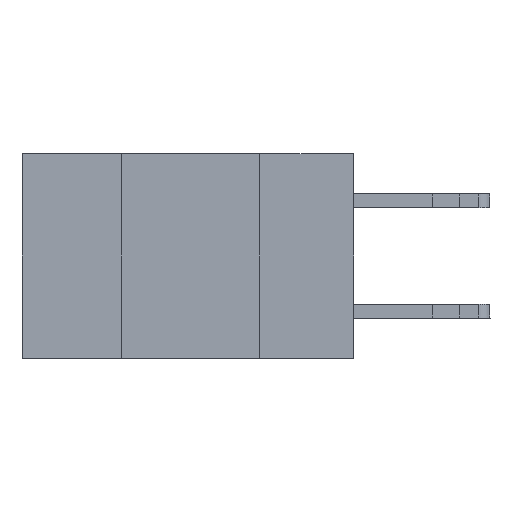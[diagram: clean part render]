
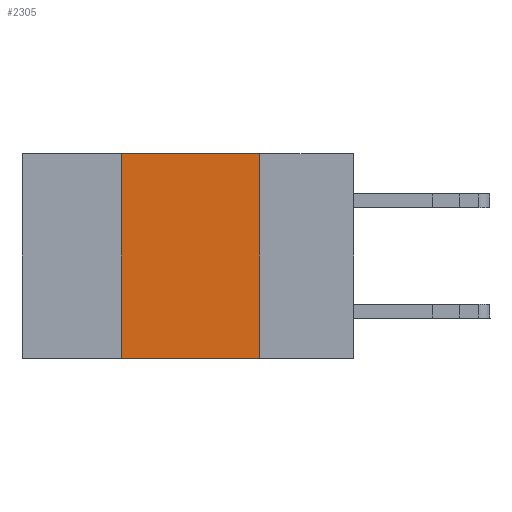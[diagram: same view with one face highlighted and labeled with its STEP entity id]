
A CAD part, left-side view. The second image highlights one B-rep face of the part: STEP entity #2305.
In plain terms, the highlighted planar face has unit normal (-1, 0, 0).
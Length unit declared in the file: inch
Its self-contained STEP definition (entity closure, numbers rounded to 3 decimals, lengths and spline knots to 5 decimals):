
#1165 = CARTESIAN_POINT ( 'NONE',  ( 0., 0.6, -0.37 ) ) ;
#1293 = ORIENTED_EDGE ( 'NONE', *, *, #8846, .F. ) ;
#1894 = VERTEX_POINT ( 'NONE', #18364 ) ;
#2266 = ORIENTED_EDGE ( 'NONE', *, *, #4004, .T. ) ;
#2305 = ADVANCED_FACE ( 'NONE', ( #12909 ), #14377, .F. ) ;
#3269 = EDGE_CURVE ( 'NONE', #5848, #14140, #14811, .T. ) ;
#3669 = ORIENTED_EDGE ( 'NONE', *, *, #13664, .F. ) ;
#4004 = EDGE_CURVE ( 'NONE', #12049, #1894, #13392, .T. ) ;
#5243 = VECTOR ( 'NONE', #10585, 39.37008 ) ;
#5584 = VECTOR ( 'NONE', #18179, 39.37008 ) ;
#5848 = VERTEX_POINT ( 'NONE', #22401 ) ;
#6698 = CARTESIAN_POINT ( 'NONE',  ( 0., 0.42, -0.37 ) ) ;
#7141 = DIRECTION ( 'NONE',  ( 0., 0., 1. ) ) ;
#7336 = CARTESIAN_POINT ( 'NONE',  ( 0., 0.17, 0. ) ) ;
#7485 = ORIENTED_EDGE ( 'NONE', *, *, #3269, .F. ) ;
#7765 = VECTOR ( 'NONE', #7141, 39.37008 ) ;
#7977 = CARTESIAN_POINT ( 'NONE',  ( 0., 0.6, 0. ) ) ;
#8846 = EDGE_CURVE ( 'NONE', #12049, #5848, #22990, .T. ) ;
#9410 = AXIS2_PLACEMENT_3D ( 'NONE', #18213, #21141, #11997 ) ;
#10585 = DIRECTION ( 'NONE',  ( 0., -1., 0. ) ) ;
#11997 = DIRECTION ( 'NONE',  ( 0., 0., -1. ) ) ;
#12049 = VERTEX_POINT ( 'NONE', #6698 ) ;
#12909 = FACE_OUTER_BOUND ( 'NONE', #15167, .T. ) ;
#13352 = DIRECTION ( 'NONE',  ( 0., -1., 0. ) ) ;
#13392 = LINE ( 'NONE', #1165, #22171 ) ;
#13664 = EDGE_CURVE ( 'NONE', #14140, #1894, #15161, .T. ) ;
#14140 = VERTEX_POINT ( 'NONE', #17716 ) ;
#14377 = PLANE ( 'NONE',  #9410 ) ;
#14811 = LINE ( 'NONE', #7977, #5243 ) ;
#15161 = LINE ( 'NONE', #7336, #5584 ) ;
#15167 = EDGE_LOOP ( 'NONE', ( #3669, #7485, #1293, #2266 ) ) ;
#17716 = CARTESIAN_POINT ( 'NONE',  ( 0., 0.17, 0. ) ) ;
#18179 = DIRECTION ( 'NONE',  ( 0., 0., -1. ) ) ;
#18213 = CARTESIAN_POINT ( 'NONE',  ( 0., 0.6, 0. ) ) ;
#18364 = CARTESIAN_POINT ( 'NONE',  ( 0., 0.17, -0.37 ) ) ;
#21141 = DIRECTION ( 'NONE',  ( 1., 0., 0. ) ) ;
#21301 = CARTESIAN_POINT ( 'NONE',  ( 0., 0.42, 0. ) ) ;
#22171 = VECTOR ( 'NONE', #13352, 39.37008 ) ;
#22401 = CARTESIAN_POINT ( 'NONE',  ( 0., 0.42, 0. ) ) ;
#22990 = LINE ( 'NONE', #21301, #7765 ) ;
